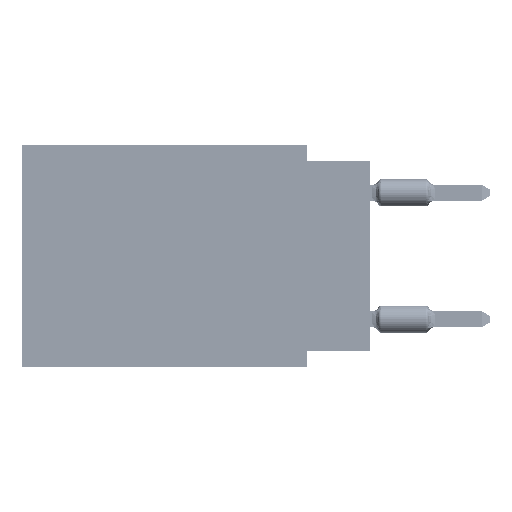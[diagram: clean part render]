
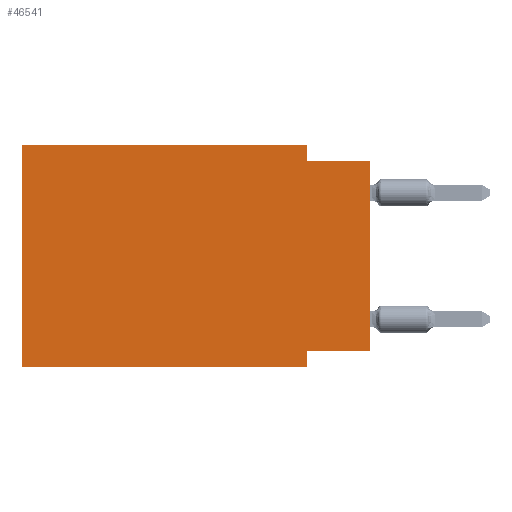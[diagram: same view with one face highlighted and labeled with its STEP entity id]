
A CAD part, left-side view. The second image highlights one B-rep face of the part: STEP entity #46541.
In plain terms, the highlighted planar face has unit normal (-1, 0, 0).
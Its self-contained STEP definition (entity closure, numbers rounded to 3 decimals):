
#358 = CARTESIAN_POINT ( 'NONE',  ( 0., 0., 0. ) ) ;
#1608 = EDGE_CURVE ( 'NONE', #25244, #69970, #43591, .T. ) ;
#1922 = LINE ( 'NONE', #10442, #29931 ) ;
#2584 = VECTOR ( 'NONE', #46236, 1000. ) ;
#2882 = AXIS2_PLACEMENT_3D ( 'NONE', #81725, #10107, #98758 ) ;
#4902 = LINE ( 'NONE', #73145, #10888 ) ;
#6647 = VECTOR ( 'NONE', #42650, 1000. ) ;
#6938 = CARTESIAN_POINT ( 'NONE',  ( 0., 2.54, -8.89 ) ) ;
#9603 = EDGE_CURVE ( 'NONE', #25244, #48906, #57451, .T. ) ;
#10107 = DIRECTION ( 'NONE',  ( 1., 0., 0. ) ) ;
#10442 = CARTESIAN_POINT ( 'NONE',  ( 0., 13.97, 0. ) ) ;
#10888 = VECTOR ( 'NONE', #74287, 1000. ) ;
#14207 = CARTESIAN_POINT ( 'NONE',  ( 0., 0., -8.255 ) ) ;
#15675 = ORIENTED_EDGE ( 'NONE', *, *, #55661, .F. ) ;
#16854 = VERTEX_POINT ( 'NONE', #54893 ) ;
#17140 = ORIENTED_EDGE ( 'NONE', *, *, #74687, .F. ) ;
#19129 = LINE ( 'NONE', #61824, #104192 ) ;
#19829 = VERTEX_POINT ( 'NONE', #65381 ) ;
#19981 = DIRECTION ( 'NONE',  ( 0., 0., 1. ) ) ;
#20533 = CARTESIAN_POINT ( 'NONE',  ( 0., 13.97, 0. ) ) ;
#22496 = VERTEX_POINT ( 'NONE', #66094 ) ;
#25244 = VERTEX_POINT ( 'NONE', #45400 ) ;
#28270 = PLANE ( 'NONE',  #2882 ) ;
#28393 = EDGE_CURVE ( 'NONE', #19829, #81237, #102000, .T. ) ;
#29153 = ORIENTED_EDGE ( 'NONE', *, *, #104890, .F. ) ;
#29918 = EDGE_LOOP ( 'NONE', ( #75227, #51265, #29153, #87493, #15675, #95208, #17140, #72309 ) ) ;
#29931 = VECTOR ( 'NONE', #79831, 1000. ) ;
#32638 = DIRECTION ( 'NONE',  ( 0., -1., 0. ) ) ;
#36220 = DIRECTION ( 'NONE',  ( 0., -1., 0. ) ) ;
#40597 = CARTESIAN_POINT ( 'NONE',  ( 0., 13.97, -8.89 ) ) ;
#41288 = VECTOR ( 'NONE', #19981, 1000. ) ;
#42650 = DIRECTION ( 'NONE',  ( 0., 0., -1. ) ) ;
#43591 = LINE ( 'NONE', #358, #81456 ) ;
#45400 = CARTESIAN_POINT ( 'NONE',  ( 0., 0., -8.255 ) ) ;
#46236 = DIRECTION ( 'NONE',  ( 0., 1., 0. ) ) ;
#46541 = ADVANCED_FACE ( 'NONE', ( #88576 ), #28270, .F. ) ;
#48906 = VERTEX_POINT ( 'NONE', #78910 ) ;
#51265 = ORIENTED_EDGE ( 'NONE', *, *, #59515, .F. ) ;
#51757 = CARTESIAN_POINT ( 'NONE',  ( 0., 2.54, -8.89 ) ) ;
#53427 = LINE ( 'NONE', #51757, #6647 ) ;
#54871 = VERTEX_POINT ( 'NONE', #64659 ) ;
#54893 = CARTESIAN_POINT ( 'NONE',  ( 0., 13.97, 0. ) ) ;
#55661 = EDGE_CURVE ( 'NONE', #19829, #16854, #81955, .T. ) ;
#57451 = LINE ( 'NONE', #14207, #2584 ) ;
#59515 = EDGE_CURVE ( 'NONE', #22496, #69970, #19129, .T. ) ;
#61824 = CARTESIAN_POINT ( 'NONE',  ( 0., 0., -0.635 ) ) ;
#64659 = CARTESIAN_POINT ( 'NONE',  ( 0., 2.54, 0. ) ) ;
#65381 = CARTESIAN_POINT ( 'NONE',  ( 0., 13.97, -8.89 ) ) ;
#66094 = CARTESIAN_POINT ( 'NONE',  ( 0., 2.54, -0.635 ) ) ;
#69248 = CARTESIAN_POINT ( 'NONE',  ( 0., 0., -0.635 ) ) ;
#69732 = DIRECTION ( 'NONE',  ( 0., 0., 1. ) ) ;
#69970 = VERTEX_POINT ( 'NONE', #69248 ) ;
#72309 = ORIENTED_EDGE ( 'NONE', *, *, #9603, .F. ) ;
#72453 = EDGE_CURVE ( 'NONE', #16854, #54871, #1922, .T. ) ;
#73145 = CARTESIAN_POINT ( 'NONE',  ( 0., 2.54, 0. ) ) ;
#74287 = DIRECTION ( 'NONE',  ( 0., 0., -1. ) ) ;
#74687 = EDGE_CURVE ( 'NONE', #48906, #81237, #53427, .T. ) ;
#75227 = ORIENTED_EDGE ( 'NONE', *, *, #1608, .T. ) ;
#78910 = CARTESIAN_POINT ( 'NONE',  ( 0., 2.54, -8.255 ) ) ;
#79831 = DIRECTION ( 'NONE',  ( 0., -1., 0. ) ) ;
#81237 = VERTEX_POINT ( 'NONE', #6938 ) ;
#81456 = VECTOR ( 'NONE', #69732, 1000. ) ;
#81725 = CARTESIAN_POINT ( 'NONE',  ( 0., 13.97, 0. ) ) ;
#81955 = LINE ( 'NONE', #20533, #41288 ) ;
#87493 = ORIENTED_EDGE ( 'NONE', *, *, #72453, .F. ) ;
#88576 = FACE_OUTER_BOUND ( 'NONE', #29918, .T. ) ;
#95208 = ORIENTED_EDGE ( 'NONE', *, *, #28393, .T. ) ;
#95430 = VECTOR ( 'NONE', #32638, 1000. ) ;
#98758 = DIRECTION ( 'NONE',  ( 0., 0., -1. ) ) ;
#102000 = LINE ( 'NONE', #40597, #95430 ) ;
#104192 = VECTOR ( 'NONE', #36220, 1000. ) ;
#104890 = EDGE_CURVE ( 'NONE', #54871, #22496, #4902, .T. ) ;
